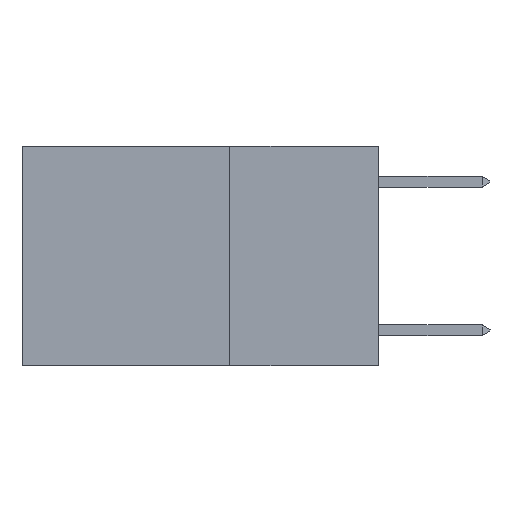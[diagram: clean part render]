
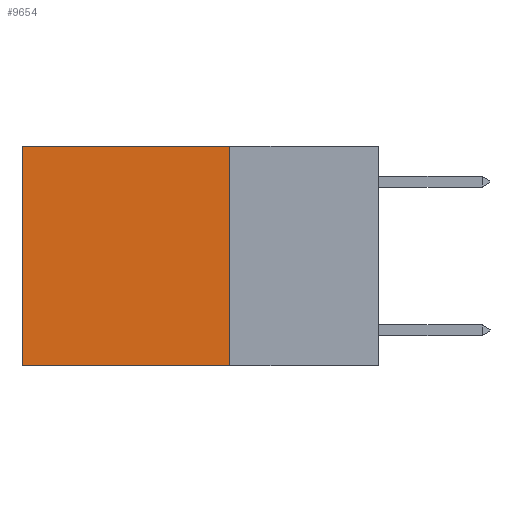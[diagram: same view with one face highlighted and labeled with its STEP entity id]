
A CAD part, left-side view. The second image highlights one B-rep face of the part: STEP entity #9654.
In plain terms, the highlighted planar face has unit normal (-1, 0, 0).
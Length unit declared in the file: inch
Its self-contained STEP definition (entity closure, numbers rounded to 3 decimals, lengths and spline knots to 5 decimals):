
#993 = CARTESIAN_POINT ( 'NONE',  ( 0.2625, 0.25, -0.37 ) ) ;
#1140 = EDGE_CURVE ( 'NONE', #2970, #4848, #1596, .T. ) ;
#1255 = VECTOR ( 'NONE', #11647, 39.37008 ) ;
#1296 = ORIENTED_EDGE ( 'NONE', *, *, #10634, .T. ) ;
#1345 = ORIENTED_EDGE ( 'NONE', *, *, #4497, .F. ) ;
#1357 = ORIENTED_EDGE ( 'NONE', *, *, #1140, .F. ) ;
#1432 = ORIENTED_EDGE ( 'NONE', *, *, #4291, .T. ) ;
#1596 = LINE ( 'NONE', #5819, #1255 ) ;
#2448 = DIRECTION ( 'NONE',  ( 0., 0., -1. ) ) ;
#2579 = DIRECTION ( 'NONE',  ( 0., 1., 0. ) ) ;
#2920 = EDGE_LOOP ( 'NONE', ( #1296, #1345, #1357, #1432 ) ) ;
#2970 = VERTEX_POINT ( 'NONE', #5729 ) ;
#3286 = CARTESIAN_POINT ( 'NONE',  ( 0.2625, 0.25, 0. ) ) ;
#4291 = EDGE_CURVE ( 'NONE', #2970, #5637, #5537, .T. ) ;
#4411 = FACE_OUTER_BOUND ( 'NONE', #2920, .T. ) ;
#4497 = EDGE_CURVE ( 'NONE', #4848, #5859, #10918, .T. ) ;
#4848 = VERTEX_POINT ( 'NONE', #993 ) ;
#5016 = DIRECTION ( 'NONE',  ( 1., 0., 0. ) ) ;
#5537 = LINE ( 'NONE', #3286, #8179 ) ;
#5546 = CARTESIAN_POINT ( 'NONE',  ( 0.2625, 0.6, 0. ) ) ;
#5637 = VERTEX_POINT ( 'NONE', #9392 ) ;
#5696 = VECTOR ( 'NONE', #2579, 39.37008 ) ;
#5729 = CARTESIAN_POINT ( 'NONE',  ( 0.2625, 0.25, 0. ) ) ;
#5819 = CARTESIAN_POINT ( 'NONE',  ( 0.2625, 0.25, 0. ) ) ;
#5859 = VERTEX_POINT ( 'NONE', #8721 ) ;
#5965 = PLANE ( 'NONE',  #6223 ) ;
#6223 = AXIS2_PLACEMENT_3D ( 'NONE', #10902, #5016, #11830 ) ;
#7633 = CARTESIAN_POINT ( 'NONE',  ( 0.2625, 0.25, -0.37 ) ) ;
#7993 = VECTOR ( 'NONE', #2448, 39.37008 ) ;
#8179 = VECTOR ( 'NONE', #12071, 39.37008 ) ;
#8721 = CARTESIAN_POINT ( 'NONE',  ( 0.2625, 0.6, -0.37 ) ) ;
#9392 = CARTESIAN_POINT ( 'NONE',  ( 0.2625, 0.6, 0. ) ) ;
#9654 = ADVANCED_FACE ( 'NONE', ( #4411 ), #5965, .F. ) ;
#10634 = EDGE_CURVE ( 'NONE', #5637, #5859, #10896, .T. ) ;
#10896 = LINE ( 'NONE', #5546, #7993 ) ;
#10902 = CARTESIAN_POINT ( 'NONE',  ( 0.2625, 0.25, 0. ) ) ;
#10918 = LINE ( 'NONE', #7633, #5696 ) ;
#11647 = DIRECTION ( 'NONE',  ( 0., 0., -1. ) ) ;
#11830 = DIRECTION ( 'NONE',  ( 0., 0., -1. ) ) ;
#12071 = DIRECTION ( 'NONE',  ( 0., 1., 0. ) ) ;
